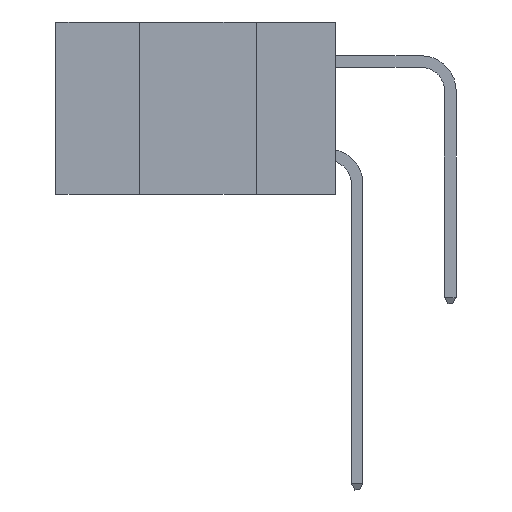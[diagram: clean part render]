
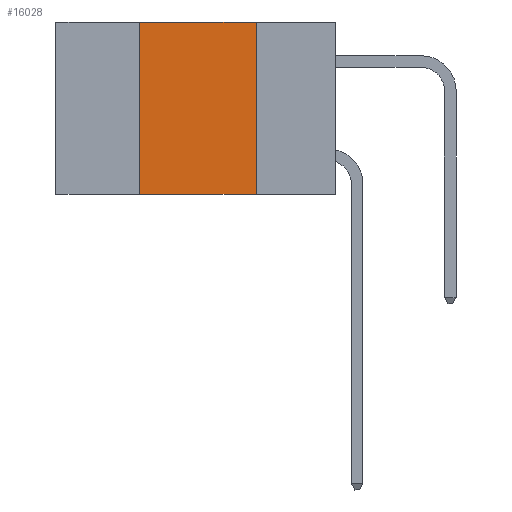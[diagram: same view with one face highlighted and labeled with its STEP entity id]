
A CAD part, left-side view. The second image highlights one B-rep face of the part: STEP entity #16028.
In plain terms, the highlighted planar face has unit normal (-1, 0, 0).
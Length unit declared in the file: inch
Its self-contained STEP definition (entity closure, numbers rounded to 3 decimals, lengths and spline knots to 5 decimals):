
#76 = LINE ( 'NONE', #9658, #8700 ) ;
#1770 = EDGE_CURVE ( 'NONE', #11406, #9611, #17146, .T. ) ;
#2071 = EDGE_CURVE ( 'NONE', #3383, #7377, #8473, .T. ) ;
#2800 = CARTESIAN_POINT ( 'NONE',  ( 0., 0.17, 0. ) ) ;
#2852 = ORIENTED_EDGE ( 'NONE', *, *, #12897, .F. ) ;
#3128 = PLANE ( 'NONE',  #4369 ) ;
#3383 = VERTEX_POINT ( 'NONE', #7692 ) ;
#4369 = AXIS2_PLACEMENT_3D ( 'NONE', #8578, #16916, #11229 ) ;
#4597 = CARTESIAN_POINT ( 'NONE',  ( 0., 0.6, -0.37 ) ) ;
#5065 = EDGE_LOOP ( 'NONE', ( #2852, #16273, #14448, #7395 ) ) ;
#6493 = CARTESIAN_POINT ( 'NONE',  ( 0., 0.6, 0. ) ) ;
#7377 = VERTEX_POINT ( 'NONE', #9415 ) ;
#7395 = ORIENTED_EDGE ( 'NONE', *, *, #2071, .T. ) ;
#7619 = DIRECTION ( 'NONE',  ( 0., -1., 0. ) ) ;
#7692 = CARTESIAN_POINT ( 'NONE',  ( 0., 0.42, -0.37 ) ) ;
#7740 = CARTESIAN_POINT ( 'NONE',  ( 0., 0.17, 0. ) ) ;
#8113 = EDGE_CURVE ( 'NONE', #3383, #11406, #76, .T. ) ;
#8269 = VECTOR ( 'NONE', #7619, 39.37008 ) ;
#8473 = LINE ( 'NONE', #4597, #8269 ) ;
#8578 = CARTESIAN_POINT ( 'NONE',  ( 0., 0.6, 0. ) ) ;
#8700 = VECTOR ( 'NONE', #11157, 39.37008 ) ;
#9415 = CARTESIAN_POINT ( 'NONE',  ( 0., 0.17, -0.37 ) ) ;
#9611 = VERTEX_POINT ( 'NONE', #2800 ) ;
#9658 = CARTESIAN_POINT ( 'NONE',  ( 0., 0.42, 0. ) ) ;
#9795 = VECTOR ( 'NONE', #17412, 39.37008 ) ;
#10205 = VECTOR ( 'NONE', #17656, 39.37008 ) ;
#11157 = DIRECTION ( 'NONE',  ( 0., 0., 1. ) ) ;
#11229 = DIRECTION ( 'NONE',  ( 0., 0., -1. ) ) ;
#11406 = VERTEX_POINT ( 'NONE', #13881 ) ;
#12897 = EDGE_CURVE ( 'NONE', #9611, #7377, #17601, .T. ) ;
#13881 = CARTESIAN_POINT ( 'NONE',  ( 0., 0.42, 0. ) ) ;
#14448 = ORIENTED_EDGE ( 'NONE', *, *, #8113, .F. ) ;
#16028 = ADVANCED_FACE ( 'NONE', ( #16836 ), #3128, .F. ) ;
#16273 = ORIENTED_EDGE ( 'NONE', *, *, #1770, .F. ) ;
#16836 = FACE_OUTER_BOUND ( 'NONE', #5065, .T. ) ;
#16916 = DIRECTION ( 'NONE',  ( 1., 0., 0. ) ) ;
#17146 = LINE ( 'NONE', #6493, #10205 ) ;
#17412 = DIRECTION ( 'NONE',  ( 0., 0., -1. ) ) ;
#17601 = LINE ( 'NONE', #7740, #9795 ) ;
#17656 = DIRECTION ( 'NONE',  ( 0., -1., 0. ) ) ;
